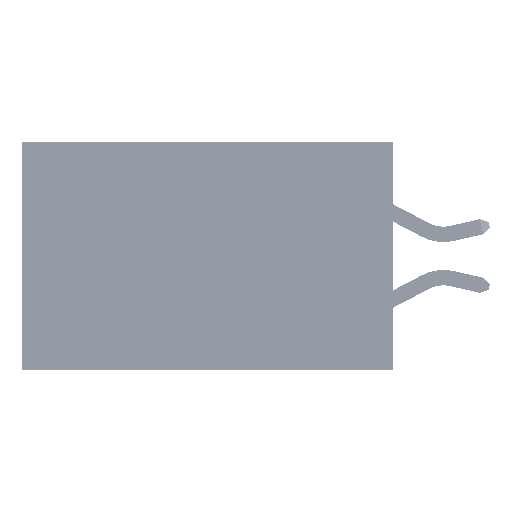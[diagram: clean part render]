
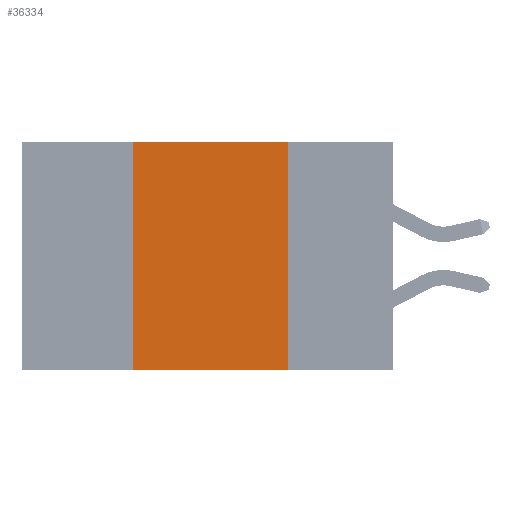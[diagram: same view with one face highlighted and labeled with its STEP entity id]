
A CAD part, left-side view. The second image highlights one B-rep face of the part: STEP entity #36334.
In plain terms, the highlighted planar face has unit normal (-1, 0, 0).
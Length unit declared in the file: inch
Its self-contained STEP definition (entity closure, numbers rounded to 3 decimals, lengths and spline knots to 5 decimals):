
#258 = VECTOR ( 'NONE', #25814, 39.37008 ) ;
#532 = VERTEX_POINT ( 'NONE', #35018 ) ;
#1516 = VERTEX_POINT ( 'NONE', #36339 ) ;
#3220 = CARTESIAN_POINT ( 'NONE',  ( 0., 0.6, -0.37 ) ) ;
#4846 = VECTOR ( 'NONE', #30394, 39.37008 ) ;
#5701 = CARTESIAN_POINT ( 'NONE',  ( 0., 0.42, -0.37 ) ) ;
#5722 = VECTOR ( 'NONE', #24657, 39.37008 ) ;
#6077 = FACE_OUTER_BOUND ( 'NONE', #25312, .T. ) ;
#7199 = PLANE ( 'NONE',  #8980 ) ;
#8009 = CARTESIAN_POINT ( 'NONE',  ( 0., 0.17, 0. ) ) ;
#8583 = EDGE_CURVE ( 'NONE', #44600, #532, #22771, .T. ) ;
#8980 = AXIS2_PLACEMENT_3D ( 'NONE', #32197, #35760, #14464 ) ;
#10425 = ORIENTED_EDGE ( 'NONE', *, *, #12533, .F. ) ;
#11467 = DIRECTION ( 'NONE',  ( 0., -1., 0. ) ) ;
#12500 = CARTESIAN_POINT ( 'NONE',  ( 0., 0.42, 0. ) ) ;
#12533 = EDGE_CURVE ( 'NONE', #1516, #22799, #28832, .T. ) ;
#14401 = ORIENTED_EDGE ( 'NONE', *, *, #8583, .F. ) ;
#14464 = DIRECTION ( 'NONE',  ( 0., 0., -1. ) ) ;
#15326 = LINE ( 'NONE', #3220, #5722 ) ;
#20396 = EDGE_CURVE ( 'NONE', #532, #1516, #43976, .T. ) ;
#22771 = LINE ( 'NONE', #12500, #4846 ) ;
#22799 = VERTEX_POINT ( 'NONE', #32916 ) ;
#24657 = DIRECTION ( 'NONE',  ( 0., -1., 0. ) ) ;
#25312 = EDGE_LOOP ( 'NONE', ( #10425, #31618, #14401, #44944 ) ) ;
#25814 = DIRECTION ( 'NONE',  ( 0., 0., -1. ) ) ;
#28832 = LINE ( 'NONE', #8009, #258 ) ;
#30394 = DIRECTION ( 'NONE',  ( 0., 0., 1. ) ) ;
#31618 = ORIENTED_EDGE ( 'NONE', *, *, #20396, .F. ) ;
#32197 = CARTESIAN_POINT ( 'NONE',  ( 0., 0.6, 0. ) ) ;
#32916 = CARTESIAN_POINT ( 'NONE',  ( 0., 0.17, -0.37 ) ) ;
#33436 = VECTOR ( 'NONE', #11467, 39.37008 ) ;
#35018 = CARTESIAN_POINT ( 'NONE',  ( 0., 0.42, 0. ) ) ;
#35760 = DIRECTION ( 'NONE',  ( 1., 0., 0. ) ) ;
#36334 = ADVANCED_FACE ( 'NONE', ( #6077 ), #7199, .F. ) ;
#36339 = CARTESIAN_POINT ( 'NONE',  ( 0., 0.17, 0. ) ) ;
#39926 = CARTESIAN_POINT ( 'NONE',  ( 0., 0.6, 0. ) ) ;
#40520 = EDGE_CURVE ( 'NONE', #44600, #22799, #15326, .T. ) ;
#43976 = LINE ( 'NONE', #39926, #33436 ) ;
#44600 = VERTEX_POINT ( 'NONE', #5701 ) ;
#44944 = ORIENTED_EDGE ( 'NONE', *, *, #40520, .T. ) ;
